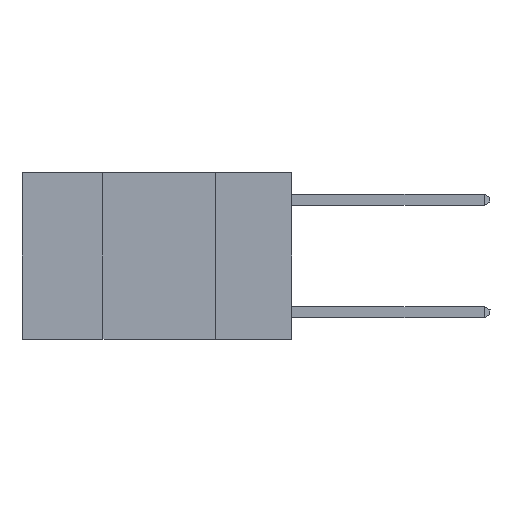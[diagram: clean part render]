
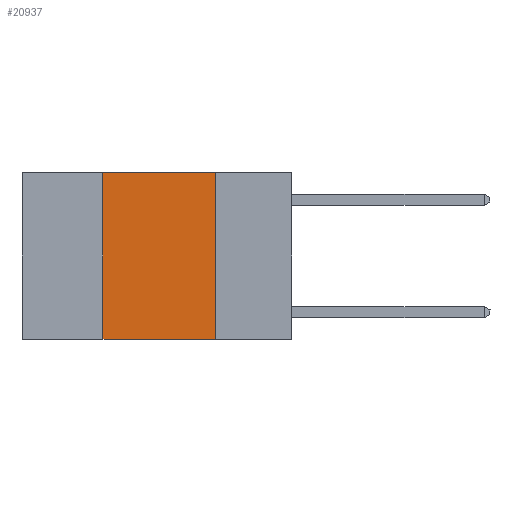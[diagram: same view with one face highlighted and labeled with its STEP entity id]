
A CAD part, left-side view. The second image highlights one B-rep face of the part: STEP entity #20937.
In plain terms, the highlighted planar face has unit normal (-1, 0, 0).
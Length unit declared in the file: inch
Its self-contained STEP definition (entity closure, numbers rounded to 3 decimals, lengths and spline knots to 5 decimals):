
#1481 = VECTOR ( 'NONE', #16605, 39.37008 ) ;
#1594 = DIRECTION ( 'NONE',  ( 0., -1., 0. ) ) ;
#2220 = CARTESIAN_POINT ( 'NONE',  ( 0., 0.42, -0.37 ) ) ;
#2335 = DIRECTION ( 'NONE',  ( 0., 0., -1. ) ) ;
#3055 = VECTOR ( 'NONE', #19694, 39.37008 ) ;
#4116 = CARTESIAN_POINT ( 'NONE',  ( 0., 0.17, 0. ) ) ;
#4534 = ORIENTED_EDGE ( 'NONE', *, *, #21740, .F. ) ;
#4610 = ORIENTED_EDGE ( 'NONE', *, *, #20545, .F. ) ;
#4659 = ORIENTED_EDGE ( 'NONE', *, *, #19527, .F. ) ;
#4735 = LINE ( 'NONE', #12821, #3055 ) ;
#5069 = ORIENTED_EDGE ( 'NONE', *, *, #16086, .T. ) ;
#6581 = CARTESIAN_POINT ( 'NONE',  ( 0., 0.42, 0. ) ) ;
#7964 = PLANE ( 'NONE',  #19644 ) ;
#9370 = VERTEX_POINT ( 'NONE', #17400 ) ;
#9760 = DIRECTION ( 'NONE',  ( 1., 0., 0. ) ) ;
#11975 = VERTEX_POINT ( 'NONE', #6581 ) ;
#12821 = CARTESIAN_POINT ( 'NONE',  ( 0., 0.6, -0.37 ) ) ;
#13035 = EDGE_LOOP ( 'NONE', ( #4534, #4610, #4659, #5069 ) ) ;
#13368 = CARTESIAN_POINT ( 'NONE',  ( 0., 0.17, 0. ) ) ;
#13970 = CARTESIAN_POINT ( 'NONE',  ( 0., 0.6, 0. ) ) ;
#14491 = VECTOR ( 'NONE', #2335, 39.37008 ) ;
#14865 = CARTESIAN_POINT ( 'NONE',  ( 0., 0.42, 0. ) ) ;
#15031 = LINE ( 'NONE', #14865, #1481 ) ;
#16086 = EDGE_CURVE ( 'NONE', #22406, #9370, #4735, .T. ) ;
#16605 = DIRECTION ( 'NONE',  ( 0., 0., 1. ) ) ;
#17400 = CARTESIAN_POINT ( 'NONE',  ( 0., 0.17, -0.37 ) ) ;
#17724 = FACE_OUTER_BOUND ( 'NONE', #13035, .T. ) ;
#17742 = VECTOR ( 'NONE', #1594, 39.37008 ) ;
#18411 = CARTESIAN_POINT ( 'NONE',  ( 0., 0.6, 0. ) ) ;
#18531 = LINE ( 'NONE', #4116, #14491 ) ;
#19005 = LINE ( 'NONE', #13970, #17742 ) ;
#19527 = EDGE_CURVE ( 'NONE', #22406, #11975, #15031, .T. ) ;
#19644 = AXIS2_PLACEMENT_3D ( 'NONE', #18411, #9760, #21756 ) ;
#19694 = DIRECTION ( 'NONE',  ( 0., -1., 0. ) ) ;
#20545 = EDGE_CURVE ( 'NONE', #11975, #21919, #19005, .T. ) ;
#20937 = ADVANCED_FACE ( 'NONE', ( #17724 ), #7964, .F. ) ;
#21740 = EDGE_CURVE ( 'NONE', #21919, #9370, #18531, .T. ) ;
#21756 = DIRECTION ( 'NONE',  ( 0., 0., -1. ) ) ;
#21919 = VERTEX_POINT ( 'NONE', #13368 ) ;
#22406 = VERTEX_POINT ( 'NONE', #2220 ) ;
